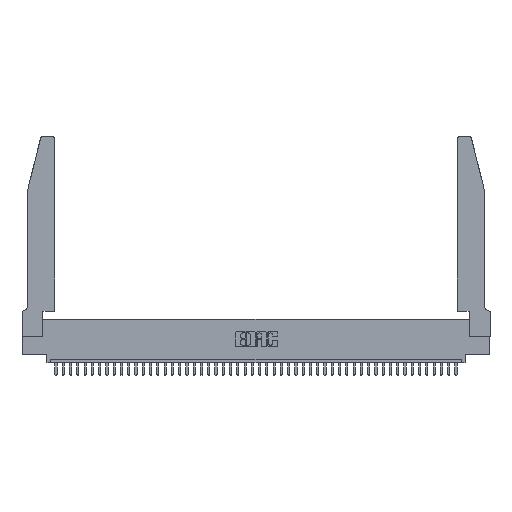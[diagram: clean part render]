
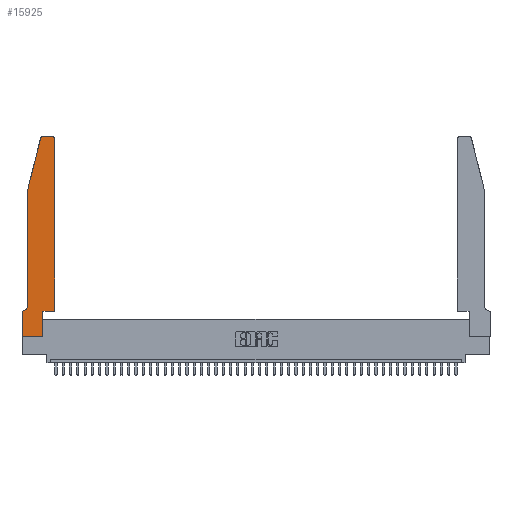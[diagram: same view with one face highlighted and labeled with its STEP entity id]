
A CAD part, top view. The second image highlights one B-rep face of the part: STEP entity #15925.
In plain terms, the highlighted planar face has unit normal (0, 0, 1).
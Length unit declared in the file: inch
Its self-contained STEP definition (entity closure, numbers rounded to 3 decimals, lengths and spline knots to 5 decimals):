
#128 = ORIENTED_EDGE ( 'NONE', *, *, #7427, .T. ) ;
#161 = ORIENTED_EDGE ( 'NONE', *, *, #31951, .T. ) ;
#714 = EDGE_CURVE ( 'NONE', #39561, #8309, #37796, .T. ) ;
#767 = ORIENTED_EDGE ( 'NONE', *, *, #714, .T. ) ;
#1379 = CARTESIAN_POINT ( 'NONE',  ( 0.284, 2.72, 0.37 ) ) ;
#1424 = VECTOR ( 'NONE', #4188, 39.37008 ) ;
#1684 = EDGE_CURVE ( 'NONE', #36118, #20578, #44503, .T. ) ;
#1721 = DIRECTION ( 'NONE',  ( 1., 0., 0. ) ) ;
#1750 = CARTESIAN_POINT ( 'NONE',  ( 0.4505, 2.72, 0.37 ) ) ;
#1856 = ORIENTED_EDGE ( 'NONE', *, *, #12662, .T. ) ;
#3058 = CARTESIAN_POINT ( 'NONE',  ( 0., 0., 0.37 ) ) ;
#4188 = DIRECTION ( 'NONE',  ( -0.239, -0.971, 0. ) ) ;
#4494 = CARTESIAN_POINT ( 'NONE',  ( 0.2865, 0.35, 0.37 ) ) ;
#5197 = AXIS2_PLACEMENT_3D ( 'NONE', #22676, #26348, #1721 ) ;
#5390 = EDGE_CURVE ( 'NONE', #29587, #26773, #23364, .T. ) ;
#7427 = EDGE_CURVE ( 'NONE', #26773, #42863, #24807, .T. ) ;
#7698 = EDGE_CURVE ( 'NONE', #20578, #19103, #42631, .T. ) ;
#7805 = DIRECTION ( 'NONE',  ( 1., 0., 0. ) ) ;
#8202 = DIRECTION ( 'NONE',  ( 0., 1., 0. ) ) ;
#8309 = VERTEX_POINT ( 'NONE', #14173 ) ;
#8371 = CARTESIAN_POINT ( 'NONE',  ( 0.4505, 0.35, 0.37 ) ) ;
#8431 = DIRECTION ( 'NONE',  ( 0., 0., 1. ) ) ;
#8610 = PLANE ( 'NONE',  #5197 ) ;
#8745 = CARTESIAN_POINT ( 'NONE',  ( 0., 0., 0.37 ) ) ;
#9569 = LINE ( 'NONE', #40562, #10655 ) ;
#9675 = CARTESIAN_POINT ( 'NONE',  ( 0.2865, 0., 0.37 ) ) ;
#10655 = VECTOR ( 'NONE', #12796, 39.37008 ) ;
#10911 = ORIENTED_EDGE ( 'NONE', *, *, #22335, .T. ) ;
#11781 = ORIENTED_EDGE ( 'NONE', *, *, #14509, .T. ) ;
#12662 = EDGE_CURVE ( 'NONE', #40561, #29587, #16335, .T. ) ;
#12796 = DIRECTION ( 'NONE',  ( -1., 0., 0. ) ) ;
#12833 = VECTOR ( 'NONE', #31331, 39.37008 ) ;
#13508 = CARTESIAN_POINT ( 'NONE',  ( 0.25487, 2.72718, 0.37 ) ) ;
#13603 = VERTEX_POINT ( 'NONE', #44379 ) ;
#14173 = CARTESIAN_POINT ( 'NONE',  ( 0.4505, 0.35, 0.37 ) ) ;
#14509 = EDGE_CURVE ( 'NONE', #43383, #40561, #9569, .T. ) ;
#15925 = ADVANCED_FACE ( 'NONE', ( #27518 ), #8610, .T. ) ;
#16335 = CIRCLE ( 'NONE', #32008, 0.03 ) ;
#16381 = CARTESIAN_POINT ( 'NONE',  ( 0.4205, 2.75, 0.37 ) ) ;
#17618 = CIRCLE ( 'NONE', #44980, 0.07 ) ;
#18638 = VECTOR ( 'NONE', #7805, 39.37008 ) ;
#19103 = VERTEX_POINT ( 'NONE', #9675 ) ;
#19667 = VECTOR ( 'NONE', #34487, 39.37008 ) ;
#19975 = DIRECTION ( 'NONE',  ( -1., 0., 0. ) ) ;
#20478 = LINE ( 'NONE', #8371, #24265 ) ;
#20578 = VERTEX_POINT ( 'NONE', #43085 ) ;
#21253 = DIRECTION ( 'NONE',  ( -1., 0., 0. ) ) ;
#21474 = CARTESIAN_POINT ( 'NONE',  ( 0.0755, 2., 0.37 ) ) ;
#22335 = EDGE_CURVE ( 'NONE', #19103, #39561, #36692, .T. ) ;
#22676 = CARTESIAN_POINT ( 'NONE',  ( 0., 0.35, 0.37 ) ) ;
#22803 = DIRECTION ( 'NONE',  ( 0., -1., 0. ) ) ;
#23243 = VERTEX_POINT ( 'NONE', #1750 ) ;
#23364 = LINE ( 'NONE', #21474, #1424 ) ;
#24068 = CIRCLE ( 'NONE', #24711, 0.03 ) ;
#24265 = VECTOR ( 'NONE', #8202, 39.37008 ) ;
#24711 = AXIS2_PLACEMENT_3D ( 'NONE', #32222, #25347, #25509 ) ;
#24807 = LINE ( 'NONE', #34663, #12833 ) ;
#24898 = CARTESIAN_POINT ( 'NONE',  ( 0.0055, 0.42, 0.37 ) ) ;
#25347 = DIRECTION ( 'NONE',  ( 0., 0., 1. ) ) ;
#25378 = DIRECTION ( 'NONE',  ( 1., 0., 0. ) ) ;
#25509 = DIRECTION ( 'NONE',  ( 1., 0., 0. ) ) ;
#26348 = DIRECTION ( 'NONE',  ( 0., 0., 1. ) ) ;
#26456 = VECTOR ( 'NONE', #22803, 39.37008 ) ;
#26727 = CARTESIAN_POINT ( 'NONE',  ( 0.2865, 0.35, 0.37 ) ) ;
#26773 = VERTEX_POINT ( 'NONE', #30542 ) ;
#26853 = VECTOR ( 'NONE', #19975, 39.37008 ) ;
#27518 = FACE_OUTER_BOUND ( 'NONE', #28367, .T. ) ;
#27565 = ORIENTED_EDGE ( 'NONE', *, *, #31157, .T. ) ;
#28257 = DIRECTION ( 'NONE',  ( 0., 0., -1. ) ) ;
#28367 = EDGE_LOOP ( 'NONE', ( #11781, #1856, #30685, #128, #38403, #27565, #33192, #44960, #10911, #767, #29533, #161 ) ) ;
#29533 = ORIENTED_EDGE ( 'NONE', *, *, #38587, .T. ) ;
#29587 = VERTEX_POINT ( 'NONE', #13508 ) ;
#30542 = CARTESIAN_POINT ( 'NONE',  ( 0.0755, 2., 0.37 ) ) ;
#30685 = ORIENTED_EDGE ( 'NONE', *, *, #5390, .T. ) ;
#31157 = EDGE_CURVE ( 'NONE', #13603, #36118, #43183, .T. ) ;
#31331 = DIRECTION ( 'NONE',  ( 0., -1., 0. ) ) ;
#31951 = EDGE_CURVE ( 'NONE', #23243, #43383, #24068, .T. ) ;
#32008 = AXIS2_PLACEMENT_3D ( 'NONE', #1379, #8431, #25378 ) ;
#32222 = CARTESIAN_POINT ( 'NONE',  ( 0.4205, 2.72, 0.37 ) ) ;
#32294 = VECTOR ( 'NONE', #33716, 39.37008 ) ;
#33192 = ORIENTED_EDGE ( 'NONE', *, *, #1684, .T. ) ;
#33625 = EDGE_CURVE ( 'NONE', #42863, #13603, #17618, .T. ) ;
#33716 = DIRECTION ( 'NONE',  ( 0., 1., 0. ) ) ;
#34005 = CARTESIAN_POINT ( 'NONE',  ( 0.0755, 0.35, 0.37 ) ) ;
#34487 = DIRECTION ( 'NONE',  ( 1., 0., 0. ) ) ;
#34663 = CARTESIAN_POINT ( 'NONE',  ( 0.0755, 2., 0.37 ) ) ;
#36118 = VERTEX_POINT ( 'NONE', #42095 ) ;
#36692 = LINE ( 'NONE', #26727, #32294 ) ;
#37796 = LINE ( 'NONE', #40209, #18638 ) ;
#38403 = ORIENTED_EDGE ( 'NONE', *, *, #33625, .T. ) ;
#38514 = CARTESIAN_POINT ( 'NONE',  ( 0.284, 2.75, 0.37 ) ) ;
#38587 = EDGE_CURVE ( 'NONE', #8309, #23243, #20478, .T. ) ;
#39561 = VERTEX_POINT ( 'NONE', #4494 ) ;
#40209 = CARTESIAN_POINT ( 'NONE',  ( 0.4505, 0.35, 0.37 ) ) ;
#40561 = VERTEX_POINT ( 'NONE', #38514 ) ;
#40562 = CARTESIAN_POINT ( 'NONE',  ( 0.2605, 2.75, 0.37 ) ) ;
#41608 = CARTESIAN_POINT ( 'NONE',  ( 0.0755, 0.42, 0.37 ) ) ;
#42095 = CARTESIAN_POINT ( 'NONE',  ( 0., 0.35, 0.37 ) ) ;
#42631 = LINE ( 'NONE', #3058, #19667 ) ;
#42863 = VERTEX_POINT ( 'NONE', #41608 ) ;
#43085 = CARTESIAN_POINT ( 'NONE',  ( 0., 0., 0.37 ) ) ;
#43183 = LINE ( 'NONE', #34005, #26853 ) ;
#43383 = VERTEX_POINT ( 'NONE', #16381 ) ;
#44379 = CARTESIAN_POINT ( 'NONE',  ( 0.0055, 0.35, 0.37 ) ) ;
#44503 = LINE ( 'NONE', #8745, #26456 ) ;
#44960 = ORIENTED_EDGE ( 'NONE', *, *, #7698, .T. ) ;
#44980 = AXIS2_PLACEMENT_3D ( 'NONE', #24898, #28257, #21253 ) ;
